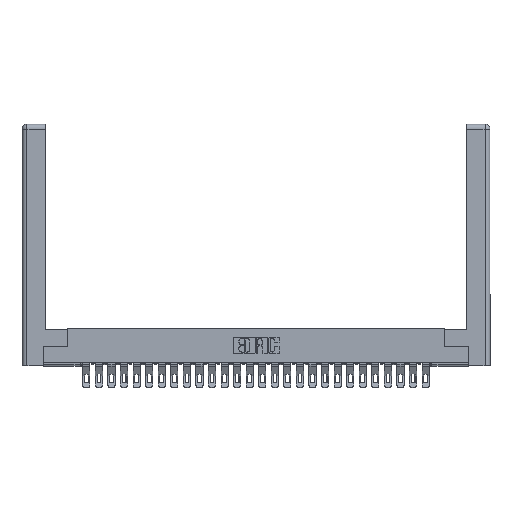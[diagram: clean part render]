
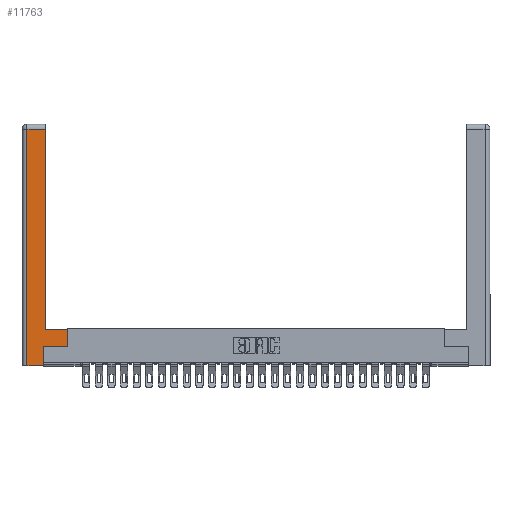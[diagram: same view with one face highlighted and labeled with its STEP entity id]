
A CAD part, top view. The second image highlights one B-rep face of the part: STEP entity #11763.
In plain terms, the highlighted planar face has unit normal (0, 0, 1).
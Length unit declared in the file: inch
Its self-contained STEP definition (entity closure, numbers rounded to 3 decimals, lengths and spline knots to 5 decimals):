
#571 = VECTOR ( 'NONE', #8564, 39.37008 ) ;
#934 = EDGE_CURVE ( 'NONE', #20522, #25710, #8131, .T. ) ;
#1075 = DIRECTION ( 'NONE',  ( -1., 0., 0. ) ) ;
#1341 = FACE_OUTER_BOUND ( 'NONE', #27446, .T. ) ;
#2051 = CARTESIAN_POINT ( 'NONE',  ( 0.265, 0., 0. ) ) ;
#2462 = CARTESIAN_POINT ( 'NONE',  ( 0.0615, 2.94, 0. ) ) ;
#4366 = DIRECTION ( 'NONE',  ( 1., 0., 0. ) ) ;
#4777 = VECTOR ( 'NONE', #7494, 39.37008 ) ;
#4824 = CARTESIAN_POINT ( 'NONE',  ( 0.565, 0.45, 0. ) ) ;
#4912 = AXIS2_PLACEMENT_3D ( 'NONE', #8011, #10555, #12790 ) ;
#5427 = VERTEX_POINT ( 'NONE', #27695 ) ;
#5454 = EDGE_CURVE ( 'NONE', #29520, #20193, #20279, .T. ) ;
#5595 = VECTOR ( 'NONE', #18543, 39.37008 ) ;
#5610 = EDGE_CURVE ( 'NONE', #12232, #29520, #17417, .T. ) ;
#5887 = VECTOR ( 'NONE', #6957, 39.37008 ) ;
#6957 = DIRECTION ( 'NONE',  ( 0., 1., 0. ) ) ;
#7494 = DIRECTION ( 'NONE',  ( 0., 1., 0. ) ) ;
#8011 = CARTESIAN_POINT ( 'NONE',  ( 0., 0., 0. ) ) ;
#8131 = LINE ( 'NONE', #16452, #5595 ) ;
#8194 = ORIENTED_EDGE ( 'NONE', *, *, #5454, .T. ) ;
#8217 = EDGE_CURVE ( 'NONE', #20193, #17489, #11528, .T. ) ;
#8564 = DIRECTION ( 'NONE',  ( 0., 1., 0. ) ) ;
#9971 = VERTEX_POINT ( 'NONE', #19040 ) ;
#10101 = CARTESIAN_POINT ( 'NONE',  ( 0.295, 0.45, 0. ) ) ;
#10425 = CARTESIAN_POINT ( 'NONE',  ( 0.0615, 0., 0. ) ) ;
#10555 = DIRECTION ( 'NONE',  ( 0., 0., -1. ) ) ;
#10569 = VECTOR ( 'NONE', #27641, 39.37008 ) ;
#11528 = LINE ( 'NONE', #14931, #29471 ) ;
#11763 = ADVANCED_FACE ( 'NONE', ( #1341 ), #17407, .F. ) ;
#12097 = ORIENTED_EDGE ( 'NONE', *, *, #29296, .T. ) ;
#12232 = VERTEX_POINT ( 'NONE', #14096 ) ;
#12571 = CARTESIAN_POINT ( 'NONE',  ( 0.265, 0.245, 0. ) ) ;
#12790 = DIRECTION ( 'NONE',  ( -1., 0., 0. ) ) ;
#14096 = CARTESIAN_POINT ( 'NONE',  ( 0.265, 0.245, 0. ) ) ;
#14931 = CARTESIAN_POINT ( 'NONE',  ( 0.295, 0.45, 0. ) ) ;
#16162 = CARTESIAN_POINT ( 'NONE',  ( 0.565, 0.45, 0. ) ) ;
#16451 = CARTESIAN_POINT ( 'NONE',  ( 0.565, 0.245, 0. ) ) ;
#16452 = CARTESIAN_POINT ( 'NONE',  ( 0.0615, 2.94, 0. ) ) ;
#16643 = LINE ( 'NONE', #2051, #19496 ) ;
#17236 = CARTESIAN_POINT ( 'NONE',  ( 0.295, 2.94, 0. ) ) ;
#17407 = PLANE ( 'NONE',  #4912 ) ;
#17417 = LINE ( 'NONE', #23423, #10569 ) ;
#17489 = VERTEX_POINT ( 'NONE', #10101 ) ;
#18300 = EDGE_CURVE ( 'NONE', #9971, #5427, #16643, .T. ) ;
#18543 = DIRECTION ( 'NONE',  ( -1., 0., 0. ) ) ;
#18885 = ORIENTED_EDGE ( 'NONE', *, *, #24769, .T. ) ;
#18911 = ORIENTED_EDGE ( 'NONE', *, *, #18300, .T. ) ;
#19040 = CARTESIAN_POINT ( 'NONE',  ( 0.0615, 0., 0. ) ) ;
#19283 = ORIENTED_EDGE ( 'NONE', *, *, #5610, .T. ) ;
#19496 = VECTOR ( 'NONE', #4366, 39.37008 ) ;
#19653 = DIRECTION ( 'NONE',  ( 0., -1., 0. ) ) ;
#20193 = VERTEX_POINT ( 'NONE', #4824 ) ;
#20279 = LINE ( 'NONE', #16162, #5887 ) ;
#20522 = VERTEX_POINT ( 'NONE', #17236 ) ;
#20960 = ORIENTED_EDGE ( 'NONE', *, *, #21954, .T. ) ;
#21954 = EDGE_CURVE ( 'NONE', #17489, #20522, #22548, .T. ) ;
#22548 = LINE ( 'NONE', #29651, #571 ) ;
#23423 = CARTESIAN_POINT ( 'NONE',  ( 0.565, 0.245, 0. ) ) ;
#24059 = VECTOR ( 'NONE', #19653, 39.37008 ) ;
#24769 = EDGE_CURVE ( 'NONE', #5427, #12232, #25294, .T. ) ;
#25294 = LINE ( 'NONE', #12571, #4777 ) ;
#25442 = ORIENTED_EDGE ( 'NONE', *, *, #8217, .T. ) ;
#25710 = VERTEX_POINT ( 'NONE', #2462 ) ;
#27446 = EDGE_LOOP ( 'NONE', ( #20960, #27655, #12097, #18911, #18885, #19283, #8194, #25442 ) ) ;
#27641 = DIRECTION ( 'NONE',  ( 1., 0., 0. ) ) ;
#27655 = ORIENTED_EDGE ( 'NONE', *, *, #934, .T. ) ;
#27695 = CARTESIAN_POINT ( 'NONE',  ( 0.265, 0., 0. ) ) ;
#29296 = EDGE_CURVE ( 'NONE', #25710, #9971, #29428, .T. ) ;
#29428 = LINE ( 'NONE', #10425, #24059 ) ;
#29471 = VECTOR ( 'NONE', #1075, 39.37008 ) ;
#29520 = VERTEX_POINT ( 'NONE', #16451 ) ;
#29651 = CARTESIAN_POINT ( 'NONE',  ( 0.295, 3., 0. ) ) ;
